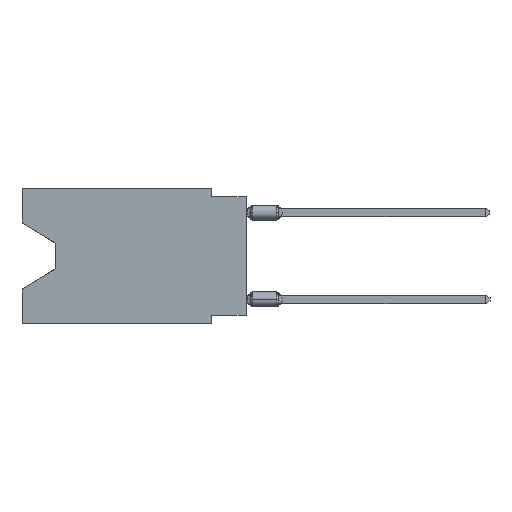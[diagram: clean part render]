
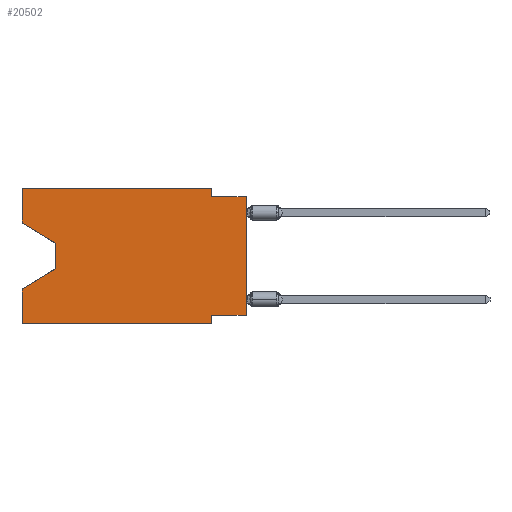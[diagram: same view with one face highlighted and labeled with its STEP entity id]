
A CAD part, left-side view. The second image highlights one B-rep face of the part: STEP entity #20502.
In plain terms, the highlighted planar face has unit normal (-1, 0, 0).
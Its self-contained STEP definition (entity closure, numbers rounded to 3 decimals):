
#1082 = ORIENTED_EDGE ( 'NONE', *, *, #3922, .F. ) ;
#1108 = CARTESIAN_POINT ( 'NONE',  ( 0., 16.383, -2.546 ) ) ;
#1140 = DIRECTION ( 'NONE',  ( 0., 0., -1. ) ) ;
#1340 = VECTOR ( 'NONE', #7615, 1000. ) ;
#1457 = DIRECTION ( 'NONE',  ( 0., 0., 1. ) ) ;
#1572 = CARTESIAN_POINT ( 'NONE',  ( 0., 0., -0.635 ) ) ;
#1605 = EDGE_LOOP ( 'NONE', ( #16446, #9016, #10672, #20303, #21626, #1082, #25843, #21873, #16777, #22305, #12950, #27859 ) ) ;
#1627 = LINE ( 'NONE', #4273, #4825 ) ;
#1758 = CARTESIAN_POINT ( 'NONE',  ( 0., 13.97, -5.893 ) ) ;
#1779 = DIRECTION ( 'NONE',  ( 0., 0., -1. ) ) ;
#1793 = CARTESIAN_POINT ( 'NONE',  ( 0., 13.97, -5.893 ) ) ;
#1826 = EDGE_CURVE ( 'NONE', #5132, #8987, #24372, .T. ) ;
#2087 = VECTOR ( 'NONE', #3062, 1000. ) ;
#2155 = CARTESIAN_POINT ( 'NONE',  ( 0., 16.383, -7.36 ) ) ;
#3062 = DIRECTION ( 'NONE',  ( 0., 0., 1. ) ) ;
#3701 = DIRECTION ( 'NONE',  ( 0., 0., 1. ) ) ;
#3794 = VECTOR ( 'NONE', #11970, 1000. ) ;
#3922 = EDGE_CURVE ( 'NONE', #22105, #18231, #29178, .T. ) ;
#4273 = CARTESIAN_POINT ( 'NONE',  ( 0., 2.54, 0. ) ) ;
#4751 = EDGE_CURVE ( 'NONE', #7094, #18917, #14080, .T. ) ;
#4825 = VECTOR ( 'NONE', #6418, 1000. ) ;
#5132 = VERTEX_POINT ( 'NONE', #1793 ) ;
#5290 = EDGE_CURVE ( 'NONE', #7439, #22105, #12818, .T. ) ;
#5447 = VERTEX_POINT ( 'NONE', #1108 ) ;
#5479 = DIRECTION ( 'NONE',  ( 0., 0., -1. ) ) ;
#6418 = DIRECTION ( 'NONE',  ( 0., 0., -1. ) ) ;
#7094 = VERTEX_POINT ( 'NONE', #25202 ) ;
#7439 = VERTEX_POINT ( 'NONE', #14867 ) ;
#7493 = CARTESIAN_POINT ( 'NONE',  ( 0., 2.54, -0.635 ) ) ;
#7615 = DIRECTION ( 'NONE',  ( 0., -1., 0. ) ) ;
#7955 = PLANE ( 'NONE',  #12573 ) ;
#8683 = DIRECTION ( 'NONE',  ( 0., 0.855, -0.519 ) ) ;
#8806 = LINE ( 'NONE', #23671, #11295 ) ;
#8987 = VERTEX_POINT ( 'NONE', #2155 ) ;
#9016 = ORIENTED_EDGE ( 'NONE', *, *, #14740, .T. ) ;
#9143 = LINE ( 'NONE', #1572, #25332 ) ;
#9988 = VERTEX_POINT ( 'NONE', #7493 ) ;
#10604 = EDGE_CURVE ( 'NONE', #9988, #26741, #9143, .T. ) ;
#10672 = ORIENTED_EDGE ( 'NONE', *, *, #1826, .T. ) ;
#11295 = VECTOR ( 'NONE', #3701, 1000. ) ;
#11970 = DIRECTION ( 'NONE',  ( 0., -0.855, -0.519 ) ) ;
#12256 = VERTEX_POINT ( 'NONE', #17094 ) ;
#12563 = CARTESIAN_POINT ( 'NONE',  ( 0., 16.383, -9.906 ) ) ;
#12573 = AXIS2_PLACEMENT_3D ( 'NONE', #28078, #18179, #5479 ) ;
#12818 = LINE ( 'NONE', #25382, #13422 ) ;
#12950 = ORIENTED_EDGE ( 'NONE', *, *, #4751, .F. ) ;
#13422 = VECTOR ( 'NONE', #25868, 1000. ) ;
#13448 = VECTOR ( 'NONE', #1779, 1000. ) ;
#13654 = LINE ( 'NONE', #31974, #21604 ) ;
#14012 = EDGE_CURVE ( 'NONE', #12256, #18231, #17516, .T. ) ;
#14080 = LINE ( 'NONE', #17048, #24934 ) ;
#14740 = EDGE_CURVE ( 'NONE', #22560, #5132, #21749, .T. ) ;
#14759 = CARTESIAN_POINT ( 'NONE',  ( 0., 16.383, -2.546 ) ) ;
#14867 = CARTESIAN_POINT ( 'NONE',  ( 0., 0., -9.271 ) ) ;
#14936 = CARTESIAN_POINT ( 'NONE',  ( 0., 16.383, 0. ) ) ;
#14984 = CARTESIAN_POINT ( 'NONE',  ( 0., 2.54, -9.906 ) ) ;
#16446 = ORIENTED_EDGE ( 'NONE', *, *, #26085, .T. ) ;
#16777 = ORIENTED_EDGE ( 'NONE', *, *, #10604, .F. ) ;
#17048 = CARTESIAN_POINT ( 'NONE',  ( 0., 16.383, 0. ) ) ;
#17094 = CARTESIAN_POINT ( 'NONE',  ( 0., 16.383, -9.906 ) ) ;
#17414 = LINE ( 'NONE', #14759, #3794 ) ;
#17516 = LINE ( 'NONE', #12563, #1340 ) ;
#17990 = CARTESIAN_POINT ( 'NONE',  ( 0., 2.54, -9.271 ) ) ;
#18179 = DIRECTION ( 'NONE',  ( 1., 0., 0. ) ) ;
#18231 = VERTEX_POINT ( 'NONE', #14984 ) ;
#18917 = VERTEX_POINT ( 'NONE', #26502 ) ;
#20303 = ORIENTED_EDGE ( 'NONE', *, *, #22937, .F. ) ;
#20502 = ADVANCED_FACE ( 'NONE', ( #30564 ), #7955, .F. ) ;
#21025 = VECTOR ( 'NONE', #8683, 1000. ) ;
#21604 = VECTOR ( 'NONE', #1457, 1000. ) ;
#21606 = CARTESIAN_POINT ( 'NONE',  ( 0., 2.54, -9.906 ) ) ;
#21626 = ORIENTED_EDGE ( 'NONE', *, *, #14012, .T. ) ;
#21749 = LINE ( 'NONE', #23906, #13448 ) ;
#21873 = ORIENTED_EDGE ( 'NONE', *, *, #24273, .T. ) ;
#22105 = VERTEX_POINT ( 'NONE', #17990 ) ;
#22305 = ORIENTED_EDGE ( 'NONE', *, *, #25499, .F. ) ;
#22560 = VERTEX_POINT ( 'NONE', #22595 ) ;
#22595 = CARTESIAN_POINT ( 'NONE',  ( 0., 13.97, -4.013 ) ) ;
#22877 = LINE ( 'NONE', #14936, #2087 ) ;
#22937 = EDGE_CURVE ( 'NONE', #12256, #8987, #22877, .T. ) ;
#23671 = CARTESIAN_POINT ( 'NONE',  ( 0., 16.383, 0. ) ) ;
#23906 = CARTESIAN_POINT ( 'NONE',  ( 0., 13.97, -4.013 ) ) ;
#24169 = DIRECTION ( 'NONE',  ( 0., -1., 0. ) ) ;
#24273 = EDGE_CURVE ( 'NONE', #7439, #26741, #13654, .T. ) ;
#24372 = LINE ( 'NONE', #1758, #21025 ) ;
#24930 = CARTESIAN_POINT ( 'NONE',  ( 0., 0., -0.635 ) ) ;
#24934 = VECTOR ( 'NONE', #24169, 1000. ) ;
#25202 = CARTESIAN_POINT ( 'NONE',  ( 0., 16.383, 0. ) ) ;
#25332 = VECTOR ( 'NONE', #29606, 1000. ) ;
#25382 = CARTESIAN_POINT ( 'NONE',  ( 0., 0., -9.271 ) ) ;
#25499 = EDGE_CURVE ( 'NONE', #18917, #9988, #1627, .T. ) ;
#25843 = ORIENTED_EDGE ( 'NONE', *, *, #5290, .F. ) ;
#25868 = DIRECTION ( 'NONE',  ( 0., 1., 0. ) ) ;
#26085 = EDGE_CURVE ( 'NONE', #5447, #22560, #17414, .T. ) ;
#26502 = CARTESIAN_POINT ( 'NONE',  ( 0., 2.54, 0. ) ) ;
#26741 = VERTEX_POINT ( 'NONE', #24930 ) ;
#27859 = ORIENTED_EDGE ( 'NONE', *, *, #30677, .F. ) ;
#28078 = CARTESIAN_POINT ( 'NONE',  ( 0., 16.383, 0. ) ) ;
#29178 = LINE ( 'NONE', #21606, #29799 ) ;
#29606 = DIRECTION ( 'NONE',  ( 0., -1., 0. ) ) ;
#29799 = VECTOR ( 'NONE', #1140, 1000. ) ;
#30564 = FACE_OUTER_BOUND ( 'NONE', #1605, .T. ) ;
#30677 = EDGE_CURVE ( 'NONE', #5447, #7094, #8806, .T. ) ;
#31974 = CARTESIAN_POINT ( 'NONE',  ( 0., 0., 0. ) ) ;
